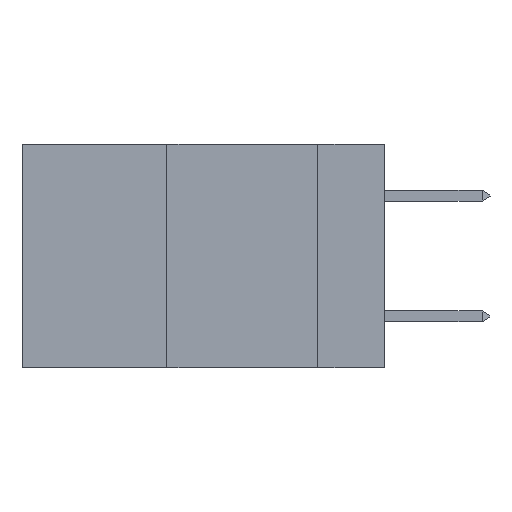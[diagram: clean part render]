
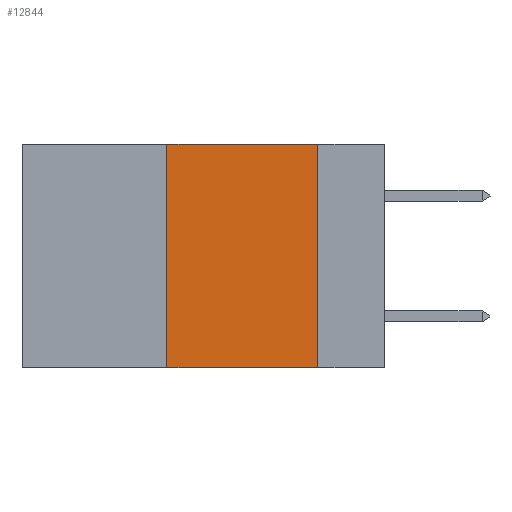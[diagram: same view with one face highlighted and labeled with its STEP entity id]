
A CAD part, left-side view. The second image highlights one B-rep face of the part: STEP entity #12844.
In plain terms, the highlighted planar face has unit normal (-1, 0, 0).
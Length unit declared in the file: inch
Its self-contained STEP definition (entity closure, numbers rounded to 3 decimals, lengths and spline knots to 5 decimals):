
#278 = CARTESIAN_POINT ( 'NONE',  ( 0., 0.6, 0. ) ) ;
#298 = CARTESIAN_POINT ( 'NONE',  ( 0., 0.11, 0. ) ) ;
#588 = VERTEX_POINT ( 'NONE', #10811 ) ;
#1713 = CARTESIAN_POINT ( 'NONE',  ( 0., 0.36, 0. ) ) ;
#2175 = EDGE_CURVE ( 'NONE', #588, #12367, #4238, .T. ) ;
#3029 = VERTEX_POINT ( 'NONE', #12592 ) ;
#3541 = VECTOR ( 'NONE', #8325, 39.37008 ) ;
#3566 = DIRECTION ( 'NONE',  ( 0., 0., -1. ) ) ;
#3934 = VECTOR ( 'NONE', #5756, 39.37008 ) ;
#4163 = CARTESIAN_POINT ( 'NONE',  ( 0., 0.6, -0.37 ) ) ;
#4238 = LINE ( 'NONE', #4163, #3541 ) ;
#5428 = FACE_OUTER_BOUND ( 'NONE', #8397, .T. ) ;
#5756 = DIRECTION ( 'NONE',  ( 0., 0., 1. ) ) ;
#5896 = ORIENTED_EDGE ( 'NONE', *, *, #10356, .F. ) ;
#6093 = CARTESIAN_POINT ( 'NONE',  ( 0., 0.6, 0. ) ) ;
#6305 = AXIS2_PLACEMENT_3D ( 'NONE', #278, #7547, #11744 ) ;
#6425 = CARTESIAN_POINT ( 'NONE',  ( 0., 0.11, -0.37 ) ) ;
#6501 = CARTESIAN_POINT ( 'NONE',  ( 0., 0.36, 0. ) ) ;
#6591 = VERTEX_POINT ( 'NONE', #1713 ) ;
#7547 = DIRECTION ( 'NONE',  ( 1., 0., 0. ) ) ;
#8325 = DIRECTION ( 'NONE',  ( 0., -1., 0. ) ) ;
#8397 = EDGE_LOOP ( 'NONE', ( #5896, #10960, #13157, #8448 ) ) ;
#8448 = ORIENTED_EDGE ( 'NONE', *, *, #2175, .T. ) ;
#8510 = VECTOR ( 'NONE', #11197, 39.37008 ) ;
#8693 = VECTOR ( 'NONE', #3566, 39.37008 ) ;
#9615 = PLANE ( 'NONE',  #6305 ) ;
#10251 = LINE ( 'NONE', #298, #8693 ) ;
#10356 = EDGE_CURVE ( 'NONE', #3029, #12367, #10251, .T. ) ;
#10811 = CARTESIAN_POINT ( 'NONE',  ( 0., 0.36, -0.37 ) ) ;
#10960 = ORIENTED_EDGE ( 'NONE', *, *, #11735, .F. ) ;
#11197 = DIRECTION ( 'NONE',  ( 0., -1., 0. ) ) ;
#11735 = EDGE_CURVE ( 'NONE', #6591, #3029, #13234, .T. ) ;
#11744 = DIRECTION ( 'NONE',  ( 0., 0., -1. ) ) ;
#11929 = LINE ( 'NONE', #6501, #3934 ) ;
#11932 = EDGE_CURVE ( 'NONE', #588, #6591, #11929, .T. ) ;
#12367 = VERTEX_POINT ( 'NONE', #6425 ) ;
#12592 = CARTESIAN_POINT ( 'NONE',  ( 0., 0.11, 0. ) ) ;
#12844 = ADVANCED_FACE ( 'NONE', ( #5428 ), #9615, .F. ) ;
#13157 = ORIENTED_EDGE ( 'NONE', *, *, #11932, .F. ) ;
#13234 = LINE ( 'NONE', #6093, #8510 ) ;
